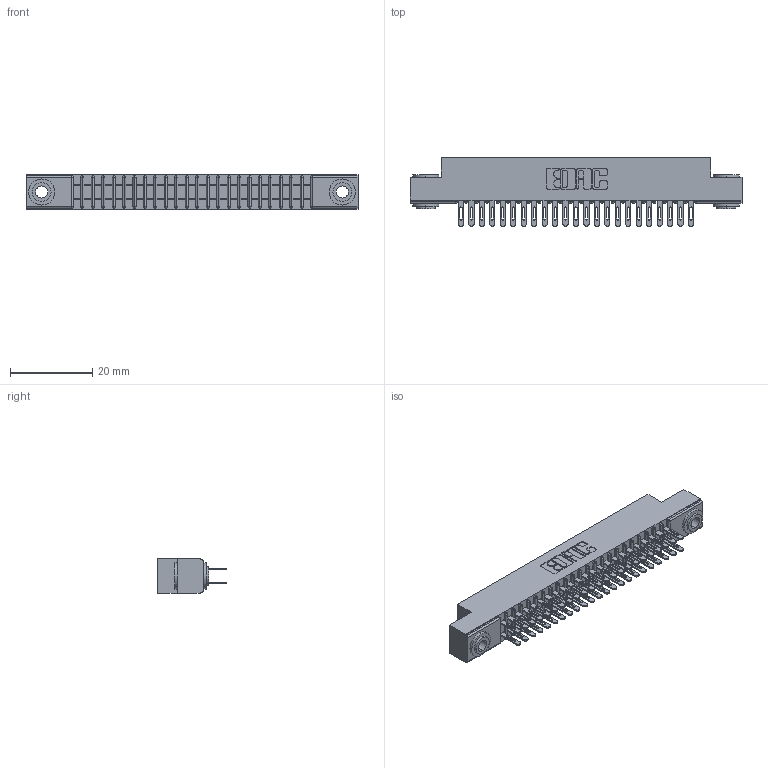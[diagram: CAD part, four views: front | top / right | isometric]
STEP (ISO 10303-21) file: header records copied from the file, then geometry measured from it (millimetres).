
FILE_DESCRIPTION (( 'STEP AP203' ), '1' );
FILE_NAME ('341-046-500-203.STEP', '2018-08-07T03:16:28', ( '' ), ( '' ), 'SwSTEP 2.0', 'SolidWorks 2016', '' );
FILE_SCHEMA (( 'CONFIG_CONTROL_DESIGN' ));
Length unit declared in the file: inch
Products named in the file (4): 341 Part_.156 (3.96) Dia Mounting Holes; 341-292-001_341-292-100; 345-250-002_345-250-002-102; 341-046-500-203
Assembly tree (49 placements, depth 2):
  341-046-500-203
    341 Part_.156 (3.96) Dia Mounting Holes
    341-292-001_341-292-100  x46
    345-250-002_345-250-002-102  x2
Bounding box: 80.64 x 16.69 x 8.38 mm (x, y, z)
Volume: 4649.2 mm3; surface area: 10353.8 mm2
Topology: 49 solids, 49 shells, 3204 faces, 9237 edges, 5982 vertices
Faces by surface type: plane 1840, cylinder 1264, sphere 48, torus 44, cone 8
Entity records: 31439 total; most frequent: CARTESIAN_POINT 5206, ORIENTED_EDGE 5162, DIRECTION 5085, EDGE_CURVE 2581, VECTOR 2051, LINE 2051, VERTEX_POINT 1638, AXIS2_PLACEMENT_3D 1517
